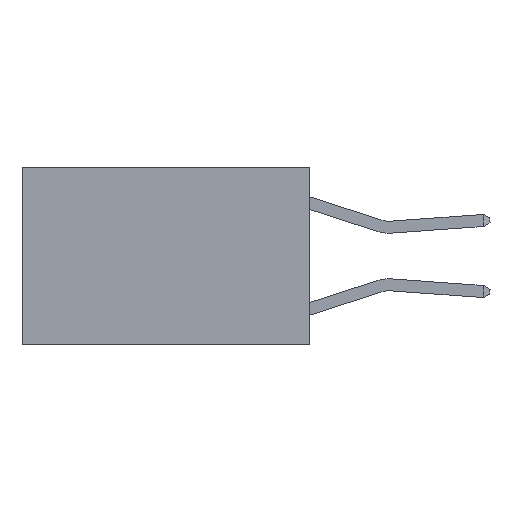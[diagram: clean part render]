
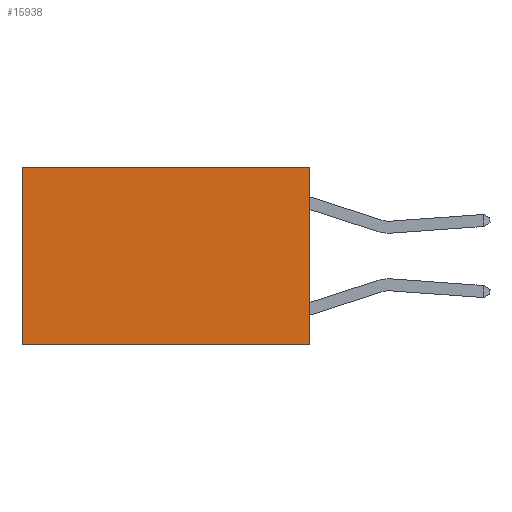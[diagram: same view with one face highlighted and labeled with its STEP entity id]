
A CAD part, left-side view. The second image highlights one B-rep face of the part: STEP entity #15938.
In plain terms, the highlighted planar face has unit normal (-1, 0, 0).
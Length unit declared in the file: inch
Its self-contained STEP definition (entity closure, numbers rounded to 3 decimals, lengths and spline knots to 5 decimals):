
#489 = DIRECTION ( 'NONE',  ( 1., 0., 0. ) ) ;
#674 = VECTOR ( 'NONE', #4216, 39.37008 ) ;
#2106 = LINE ( 'NONE', #7023, #9727 ) ;
#2685 = CARTESIAN_POINT ( 'NONE',  ( 0.2625, 0., -0.37 ) ) ;
#2763 = CARTESIAN_POINT ( 'NONE',  ( 0.2625, 0.6, -0.37 ) ) ;
#2791 = CARTESIAN_POINT ( 'NONE',  ( 0.2625, 0.6, 0. ) ) ;
#2954 = FACE_OUTER_BOUND ( 'NONE', #3246, .T. ) ;
#3100 = ORIENTED_EDGE ( 'NONE', *, *, #13457, .F. ) ;
#3246 = EDGE_LOOP ( 'NONE', ( #9297, #3100, #8051, #6961 ) ) ;
#3891 = EDGE_CURVE ( 'NONE', #10686, #12277, #19477, .T. ) ;
#4177 = CARTESIAN_POINT ( 'NONE',  ( 0.2625, 0., 0. ) ) ;
#4216 = DIRECTION ( 'NONE',  ( 0., 1., 0. ) ) ;
#4934 = VECTOR ( 'NONE', #17066, 39.37008 ) ;
#5879 = VECTOR ( 'NONE', #16643, 39.37008 ) ;
#6961 = ORIENTED_EDGE ( 'NONE', *, *, #3891, .T. ) ;
#7023 = CARTESIAN_POINT ( 'NONE',  ( 0.2625, 0., 0. ) ) ;
#8051 = ORIENTED_EDGE ( 'NONE', *, *, #12690, .F. ) ;
#8061 = CARTESIAN_POINT ( 'NONE',  ( 0.2625, 0., 0. ) ) ;
#8558 = DIRECTION ( 'NONE',  ( 0., 0., -1. ) ) ;
#8596 = CARTESIAN_POINT ( 'NONE',  ( 0.2625, 0., 0. ) ) ;
#9297 = ORIENTED_EDGE ( 'NONE', *, *, #9430, .T. ) ;
#9430 = EDGE_CURVE ( 'NONE', #12277, #11425, #17326, .T. ) ;
#9631 = AXIS2_PLACEMENT_3D ( 'NONE', #8061, #489, #11178 ) ;
#9727 = VECTOR ( 'NONE', #8558, 39.37008 ) ;
#10686 = VERTEX_POINT ( 'NONE', #4177 ) ;
#11178 = DIRECTION ( 'NONE',  ( 0., 0., -1. ) ) ;
#11425 = VERTEX_POINT ( 'NONE', #2763 ) ;
#12277 = VERTEX_POINT ( 'NONE', #15461 ) ;
#12690 = EDGE_CURVE ( 'NONE', #10686, #17021, #2106, .T. ) ;
#13457 = EDGE_CURVE ( 'NONE', #17021, #11425, #17098, .T. ) ;
#15461 = CARTESIAN_POINT ( 'NONE',  ( 0.2625, 0.6, 0. ) ) ;
#15938 = ADVANCED_FACE ( 'NONE', ( #2954 ), #18978, .F. ) ;
#16643 = DIRECTION ( 'NONE',  ( 0., 0., -1. ) ) ;
#17021 = VERTEX_POINT ( 'NONE', #19009 ) ;
#17066 = DIRECTION ( 'NONE',  ( 0., 1., 0. ) ) ;
#17098 = LINE ( 'NONE', #2685, #674 ) ;
#17326 = LINE ( 'NONE', #2791, #5879 ) ;
#18978 = PLANE ( 'NONE',  #9631 ) ;
#19009 = CARTESIAN_POINT ( 'NONE',  ( 0.2625, 0., -0.37 ) ) ;
#19477 = LINE ( 'NONE', #8596, #4934 ) ;
